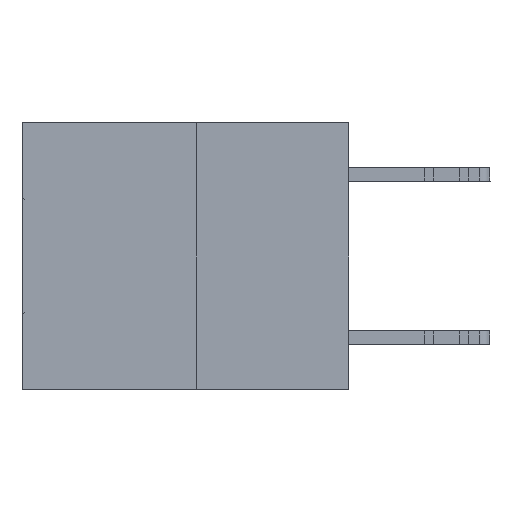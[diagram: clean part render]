
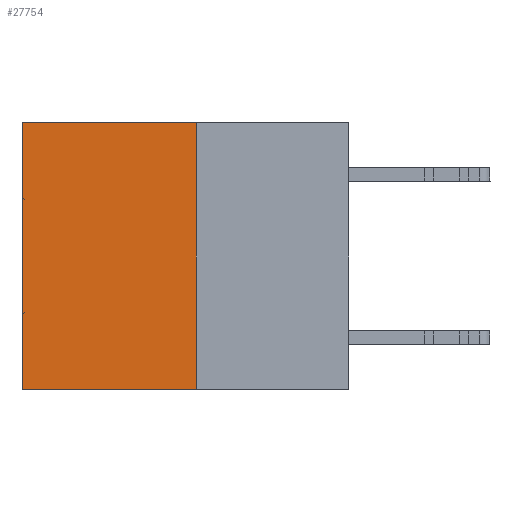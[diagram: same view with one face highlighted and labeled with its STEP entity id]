
A CAD part, left-side view. The second image highlights one B-rep face of the part: STEP entity #27754.
In plain terms, the highlighted planar face has unit normal (-1, 0, 0).
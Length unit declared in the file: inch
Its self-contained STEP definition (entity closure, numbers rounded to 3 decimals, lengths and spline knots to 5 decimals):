
#246 = LINE ( 'NONE', #5347, #6028 ) ;
#992 = ORIENTED_EDGE ( 'NONE', *, *, #16274, .T. ) ;
#1495 = EDGE_CURVE ( 'NONE', #19663, #1789, #246, .T. ) ;
#1789 = VERTEX_POINT ( 'NONE', #6118 ) ;
#1908 = CARTESIAN_POINT ( 'NONE',  ( 0.3165, 0.6, -0.49 ) ) ;
#3898 = EDGE_LOOP ( 'NONE', ( #6354, #28075, #15305, #992 ) ) ;
#4030 = CARTESIAN_POINT ( 'NONE',  ( 0.3165, 0.28, -0.49 ) ) ;
#4680 = LINE ( 'NONE', #28583, #29084 ) ;
#5347 = CARTESIAN_POINT ( 'NONE',  ( 0.3165, 0.28, -0.49 ) ) ;
#6028 = VECTOR ( 'NONE', #33613, 39.37008 ) ;
#6118 = CARTESIAN_POINT ( 'NONE',  ( 0.3165, 0.28, -0.49 ) ) ;
#6351 = CARTESIAN_POINT ( 'NONE',  ( 0.3165, 0.6, 0. ) ) ;
#6354 = ORIENTED_EDGE ( 'NONE', *, *, #30080, .T. ) ;
#6771 = CARTESIAN_POINT ( 'NONE',  ( 0.3165, 0.28, -0.49 ) ) ;
#7882 = DIRECTION ( 'NONE',  ( 0., 1., 0. ) ) ;
#10939 = EDGE_CURVE ( 'NONE', #1789, #19012, #27989, .T. ) ;
#15305 = ORIENTED_EDGE ( 'NONE', *, *, #1495, .F. ) ;
#16274 = EDGE_CURVE ( 'NONE', #19663, #27968, #4680, .T. ) ;
#19012 = VERTEX_POINT ( 'NONE', #29273 ) ;
#19663 = VERTEX_POINT ( 'NONE', #29951 ) ;
#19996 = PLANE ( 'NONE',  #30273 ) ;
#21094 = VECTOR ( 'NONE', #27567, 39.37008 ) ;
#21832 = FACE_OUTER_BOUND ( 'NONE', #3898, .T. ) ;
#22246 = DIRECTION ( 'NONE',  ( 0., 0., -1. ) ) ;
#22476 = DIRECTION ( 'NONE',  ( 1., 0., 0. ) ) ;
#22731 = DIRECTION ( 'NONE',  ( 0., 0., -1. ) ) ;
#26770 = LINE ( 'NONE', #1908, #32012 ) ;
#27567 = DIRECTION ( 'NONE',  ( 0., 1., 0. ) ) ;
#27754 = ADVANCED_FACE ( 'NONE', ( #21832 ), #19996, .F. ) ;
#27968 = VERTEX_POINT ( 'NONE', #6351 ) ;
#27989 = LINE ( 'NONE', #6771, #21094 ) ;
#28075 = ORIENTED_EDGE ( 'NONE', *, *, #10939, .F. ) ;
#28583 = CARTESIAN_POINT ( 'NONE',  ( 0.3165, 0.28, 0. ) ) ;
#29084 = VECTOR ( 'NONE', #7882, 39.37008 ) ;
#29273 = CARTESIAN_POINT ( 'NONE',  ( 0.3165, 0.6, -0.49 ) ) ;
#29951 = CARTESIAN_POINT ( 'NONE',  ( 0.3165, 0.28, 0. ) ) ;
#30080 = EDGE_CURVE ( 'NONE', #27968, #19012, #26770, .T. ) ;
#30273 = AXIS2_PLACEMENT_3D ( 'NONE', #4030, #22476, #22246 ) ;
#32012 = VECTOR ( 'NONE', #22731, 39.37008 ) ;
#33613 = DIRECTION ( 'NONE',  ( 0., 0., -1. ) ) ;
